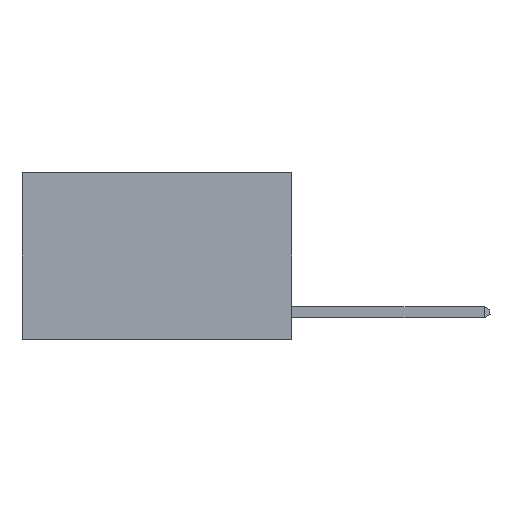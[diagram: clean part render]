
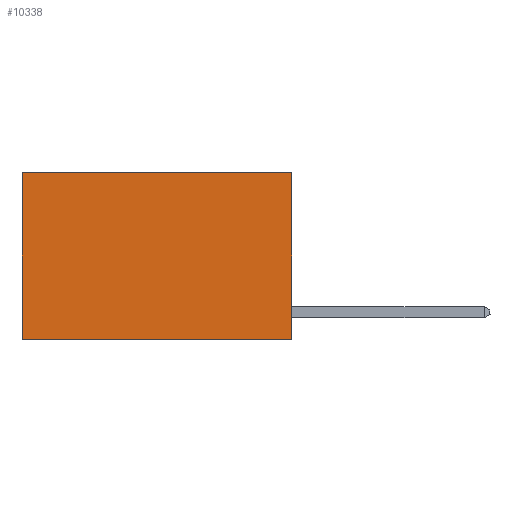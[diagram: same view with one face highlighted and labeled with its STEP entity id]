
A CAD part, left-side view. The second image highlights one B-rep face of the part: STEP entity #10338.
In plain terms, the highlighted planar face has unit normal (-1, 0, 0).
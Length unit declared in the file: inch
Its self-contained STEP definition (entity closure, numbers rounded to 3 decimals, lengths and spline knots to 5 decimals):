
#1524 = VERTEX_POINT ( 'NONE', #9989 ) ;
#1819 = CARTESIAN_POINT ( 'NONE',  ( 0.2625, 0.6, 0. ) ) ;
#1921 = VECTOR ( 'NONE', #14287, 39.37008 ) ;
#3637 = ORIENTED_EDGE ( 'NONE', *, *, #18460, .T. ) ;
#4714 = VECTOR ( 'NONE', #17899, 39.37008 ) ;
#5920 = LINE ( 'NONE', #8659, #9391 ) ;
#7183 = EDGE_CURVE ( 'NONE', #9176, #7734, #5920, .T. ) ;
#7734 = VERTEX_POINT ( 'NONE', #18509 ) ;
#7855 = LINE ( 'NONE', #7878, #18948 ) ;
#7878 = CARTESIAN_POINT ( 'NONE',  ( 0.2625, 0., -0.37 ) ) ;
#8030 = DIRECTION ( 'NONE',  ( 1., 0., 0. ) ) ;
#8441 = CARTESIAN_POINT ( 'NONE',  ( 0.2625, 0., 0. ) ) ;
#8659 = CARTESIAN_POINT ( 'NONE',  ( 0.2625, 0., 0. ) ) ;
#8920 = AXIS2_PLACEMENT_3D ( 'NONE', #15260, #8030, #18146 ) ;
#9176 = VERTEX_POINT ( 'NONE', #11562 ) ;
#9391 = VECTOR ( 'NONE', #18767, 39.37008 ) ;
#9864 = ORIENTED_EDGE ( 'NONE', *, *, #10872, .F. ) ;
#9989 = CARTESIAN_POINT ( 'NONE',  ( 0.2625, 0.6, -0.37 ) ) ;
#10142 = VERTEX_POINT ( 'NONE', #13958 ) ;
#10289 = LINE ( 'NONE', #8441, #1921 ) ;
#10338 = ADVANCED_FACE ( 'NONE', ( #12236 ), #16748, .F. ) ;
#10872 = EDGE_CURVE ( 'NONE', #10142, #1524, #7855, .T. ) ;
#11562 = CARTESIAN_POINT ( 'NONE',  ( 0.2625, 0., 0. ) ) ;
#12236 = FACE_OUTER_BOUND ( 'NONE', #18175, .T. ) ;
#12384 = ORIENTED_EDGE ( 'NONE', *, *, #13996, .F. ) ;
#13958 = CARTESIAN_POINT ( 'NONE',  ( 0.2625, 0., -0.37 ) ) ;
#13996 = EDGE_CURVE ( 'NONE', #9176, #10142, #10289, .T. ) ;
#14287 = DIRECTION ( 'NONE',  ( 0., 0., -1. ) ) ;
#15260 = CARTESIAN_POINT ( 'NONE',  ( 0.2625, 0., 0. ) ) ;
#16378 = LINE ( 'NONE', #1819, #4714 ) ;
#16608 = DIRECTION ( 'NONE',  ( 0., 1., 0. ) ) ;
#16748 = PLANE ( 'NONE',  #8920 ) ;
#17899 = DIRECTION ( 'NONE',  ( 0., 0., -1. ) ) ;
#18062 = ORIENTED_EDGE ( 'NONE', *, *, #7183, .T. ) ;
#18146 = DIRECTION ( 'NONE',  ( 0., 0., -1. ) ) ;
#18175 = EDGE_LOOP ( 'NONE', ( #3637, #9864, #12384, #18062 ) ) ;
#18460 = EDGE_CURVE ( 'NONE', #7734, #1524, #16378, .T. ) ;
#18509 = CARTESIAN_POINT ( 'NONE',  ( 0.2625, 0.6, 0. ) ) ;
#18767 = DIRECTION ( 'NONE',  ( 0., 1., 0. ) ) ;
#18948 = VECTOR ( 'NONE', #16608, 39.37008 ) ;
